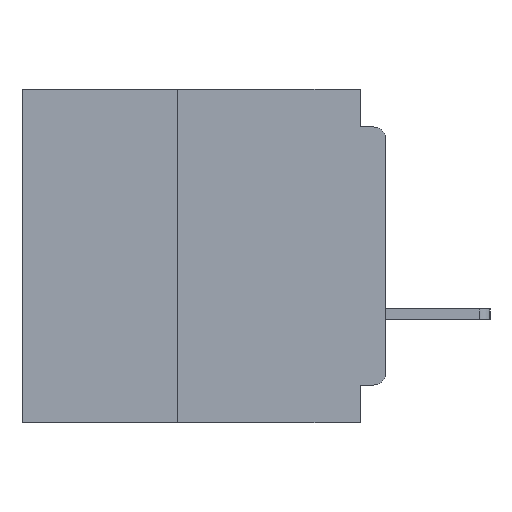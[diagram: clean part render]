
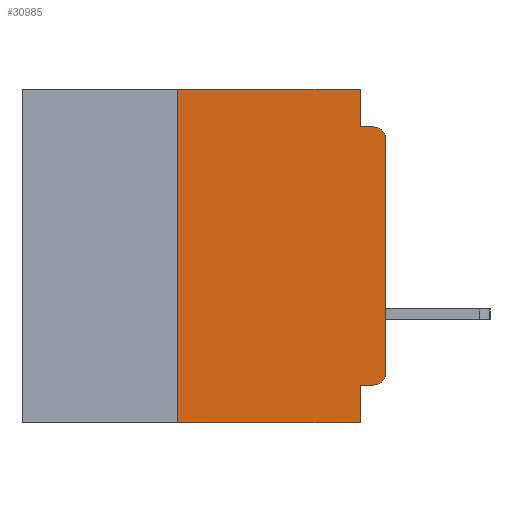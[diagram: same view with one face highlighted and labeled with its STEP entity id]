
A CAD part, left-side view. The second image highlights one B-rep face of the part: STEP entity #30985.
In plain terms, the highlighted planar face has unit normal (-1, 0, 0).
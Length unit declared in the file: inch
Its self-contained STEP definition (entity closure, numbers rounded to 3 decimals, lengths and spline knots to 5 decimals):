
#1734 = DIRECTION ( 'NONE',  ( 0., 0., 1. ) ) ;
#2814 = DIRECTION ( 'NONE',  ( 0., 0., -1. ) ) ;
#3593 = VECTOR ( 'NONE', #46212, 39.37008 ) ;
#3756 = DIRECTION ( 'NONE',  ( 0., -1., 0. ) ) ;
#4483 = CARTESIAN_POINT ( 'NONE',  ( 0., 0.015, -0.06 ) ) ;
#4509 = VECTOR ( 'NONE', #1734, 39.37008 ) ;
#4787 = LINE ( 'NONE', #27731, #3593 ) ;
#5431 = LINE ( 'NONE', #29711, #42771 ) ;
#6771 = CARTESIAN_POINT ( 'NONE',  ( 0., 0.437, 0. ) ) ;
#6774 = VECTOR ( 'NONE', #38751, 39.37008 ) ;
#6997 = VECTOR ( 'NONE', #3756, 39.37008 ) ;
#8220 = AXIS2_PLACEMENT_3D ( 'NONE', #47497, #25241, #2814 ) ;
#8235 = DIRECTION ( 'NONE',  ( 0., 0., -1. ) ) ;
#9235 = VERTEX_POINT ( 'NONE', #47083 ) ;
#10698 = DIRECTION ( 'NONE',  ( 1., 0., 0. ) ) ;
#11623 = EDGE_LOOP ( 'NONE', ( #19061, #19817, #22426, #24103, #24985, #25484, #30964, #31704, #33038, #36622 ) ) ;
#12223 = EDGE_CURVE ( 'NONE', #32061, #9235, #28750, .T. ) ;
#12658 = CARTESIAN_POINT ( 'NONE',  ( 0., 0., 0. ) ) ;
#12689 = CARTESIAN_POINT ( 'NONE',  ( 0., 0.031, -0.4 ) ) ;
#14390 = EDGE_CURVE ( 'NONE', #21241, #15629, #40690, .T. ) ;
#15629 = VERTEX_POINT ( 'NONE', #39152 ) ;
#15784 = CARTESIAN_POINT ( 'NONE',  ( 0., 0.031, -0.355 ) ) ;
#16504 = DIRECTION ( 'NONE',  ( 0., 1., 0. ) ) ;
#17343 = VERTEX_POINT ( 'NONE', #46074 ) ;
#17529 = AXIS2_PLACEMENT_3D ( 'NONE', #6771, #10698, #36829 ) ;
#19061 = ORIENTED_EDGE ( 'NONE', *, *, #21322, .T. ) ;
#19773 = VECTOR ( 'NONE', #42495, 39.37008 ) ;
#19817 = ORIENTED_EDGE ( 'NONE', *, *, #12223, .T. ) ;
#20844 = VERTEX_POINT ( 'NONE', #35422 ) ;
#21241 = VERTEX_POINT ( 'NONE', #15784 ) ;
#21322 = EDGE_CURVE ( 'NONE', #30149, #32061, #35469, .T. ) ;
#22336 = EDGE_CURVE ( 'NONE', #17343, #29560, #35681, .T. ) ;
#22426 = ORIENTED_EDGE ( 'NONE', *, *, #42190, .F. ) ;
#23748 = VERTEX_POINT ( 'NONE', #34452 ) ;
#24103 = ORIENTED_EDGE ( 'NONE', *, *, #34440, .F. ) ;
#24755 = EDGE_CURVE ( 'NONE', #42350, #21241, #33659, .T. ) ;
#24985 = ORIENTED_EDGE ( 'NONE', *, *, #22336, .F. ) ;
#25241 = DIRECTION ( 'NONE',  ( -1., 0., 0. ) ) ;
#25484 = ORIENTED_EDGE ( 'NONE', *, *, #31923, .F. ) ;
#25722 = VECTOR ( 'NONE', #40833, 39.37008 ) ;
#25875 = CARTESIAN_POINT ( 'NONE',  ( 0., 0.437, 0. ) ) ;
#26200 = CARTESIAN_POINT ( 'NONE',  ( 0., 0., -0.045 ) ) ;
#26893 = EDGE_CURVE ( 'NONE', #20844, #15629, #5431, .T. ) ;
#27731 = CARTESIAN_POINT ( 'NONE',  ( 0., 0.031, 0. ) ) ;
#28019 = AXIS2_PLACEMENT_3D ( 'NONE', #4483, #30682, #8235 ) ;
#28750 = CIRCLE ( 'NONE', #28019, 0.015 ) ;
#29354 = PLANE ( 'NONE',  #17529 ) ;
#29560 = VERTEX_POINT ( 'NONE', #32544 ) ;
#29711 = CARTESIAN_POINT ( 'NONE',  ( 0., 0.437, -0.4 ) ) ;
#30149 = VERTEX_POINT ( 'NONE', #43087 ) ;
#30682 = DIRECTION ( 'NONE',  ( -1., 0., 0. ) ) ;
#30964 = ORIENTED_EDGE ( 'NONE', *, *, #26893, .T. ) ;
#30985 = ADVANCED_FACE ( 'NONE', ( #38441 ), #29354, .F. ) ;
#31704 = ORIENTED_EDGE ( 'NONE', *, *, #14390, .F. ) ;
#31923 = EDGE_CURVE ( 'NONE', #20844, #17343, #34392, .T. ) ;
#32061 = VERTEX_POINT ( 'NONE', #39657 ) ;
#32544 = CARTESIAN_POINT ( 'NONE',  ( 0., 0.031, 0. ) ) ;
#33038 = ORIENTED_EDGE ( 'NONE', *, *, #24755, .F. ) ;
#33659 = LINE ( 'NONE', #38827, #42330 ) ;
#34392 = LINE ( 'NONE', #46450, #4509 ) ;
#34440 = EDGE_CURVE ( 'NONE', #29560, #23748, #4787, .T. ) ;
#34452 = CARTESIAN_POINT ( 'NONE',  ( 0., 0.031, -0.045 ) ) ;
#35422 = CARTESIAN_POINT ( 'NONE',  ( 0., 0.25, -0.4 ) ) ;
#35469 = LINE ( 'NONE', #12658, #6774 ) ;
#35681 = LINE ( 'NONE', #25875, #25722 ) ;
#35691 = LINE ( 'NONE', #26200, #6997 ) ;
#36622 = ORIENTED_EDGE ( 'NONE', *, *, #45603, .T. ) ;
#36829 = DIRECTION ( 'NONE',  ( 0., 0., -1. ) ) ;
#38381 = CARTESIAN_POINT ( 'NONE',  ( 0., 0.015, -0.355 ) ) ;
#38410 = CIRCLE ( 'NONE', #8220, 0.015 ) ;
#38441 = FACE_OUTER_BOUND ( 'NONE', #11623, .T. ) ;
#38751 = DIRECTION ( 'NONE',  ( 0., 0., 1. ) ) ;
#38827 = CARTESIAN_POINT ( 'NONE',  ( 0., 0., -0.355 ) ) ;
#39152 = CARTESIAN_POINT ( 'NONE',  ( 0., 0.031, -0.4 ) ) ;
#39657 = CARTESIAN_POINT ( 'NONE',  ( 0., 0., -0.06 ) ) ;
#40690 = LINE ( 'NONE', #12689, #19773 ) ;
#40833 = DIRECTION ( 'NONE',  ( 0., -1., 0. ) ) ;
#40887 = DIRECTION ( 'NONE',  ( 0., -1., 0. ) ) ;
#42190 = EDGE_CURVE ( 'NONE', #23748, #9235, #35691, .T. ) ;
#42330 = VECTOR ( 'NONE', #16504, 39.37008 ) ;
#42350 = VERTEX_POINT ( 'NONE', #38381 ) ;
#42495 = DIRECTION ( 'NONE',  ( 0., 0., -1. ) ) ;
#42771 = VECTOR ( 'NONE', #40887, 39.37008 ) ;
#43087 = CARTESIAN_POINT ( 'NONE',  ( 0., 0., -0.34 ) ) ;
#45603 = EDGE_CURVE ( 'NONE', #42350, #30149, #38410, .T. ) ;
#46074 = CARTESIAN_POINT ( 'NONE',  ( 0., 0.25, 0. ) ) ;
#46212 = DIRECTION ( 'NONE',  ( 0., 0., -1. ) ) ;
#46450 = CARTESIAN_POINT ( 'NONE',  ( 0., 0.25, -0.4 ) ) ;
#47083 = CARTESIAN_POINT ( 'NONE',  ( 0., 0.015, -0.045 ) ) ;
#47497 = CARTESIAN_POINT ( 'NONE',  ( 0., 0.015, -0.34 ) ) ;
